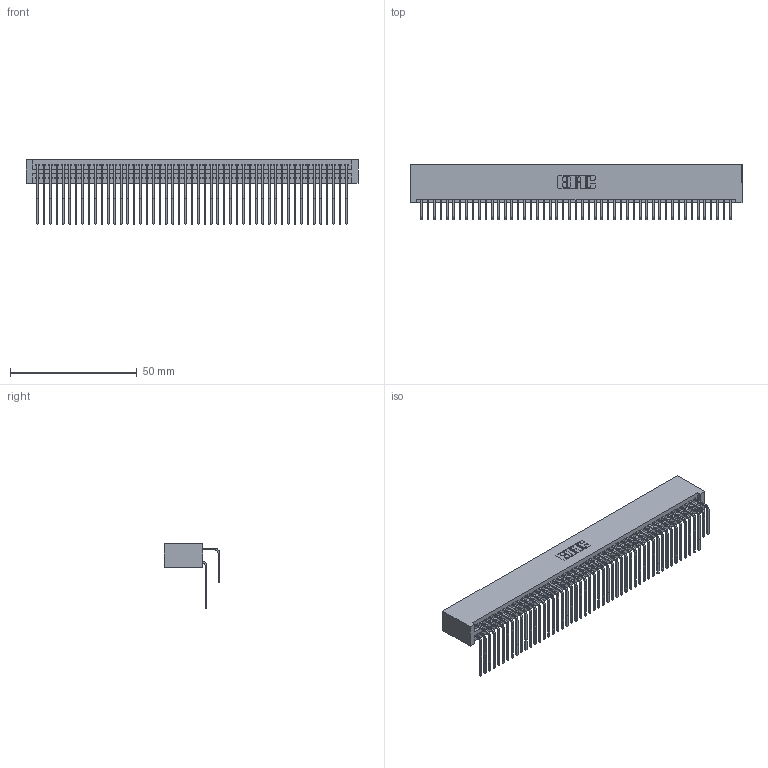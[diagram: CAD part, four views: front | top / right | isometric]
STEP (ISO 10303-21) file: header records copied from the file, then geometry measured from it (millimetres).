
FILE_DESCRIPTION (( 'STEP AP203' ), '1' );
FILE_NAME ('345-098-558-201.STEP', '2019-11-02T12:53:45', ( '' ), ( '' ), 'SwSTEP 2.0', 'SolidWorks 2016', '' );
FILE_SCHEMA (( 'CONFIG_CONTROL_DESIGN' ));
Length unit declared in the file: inch
Products named in the file (4): 345-292-001_558 Tail - 2; 345 Part_No Mounting Lugs; 345-292-001_558 559 Tail - 1; 345-098-558-201
Assembly tree (99 placements, depth 2):
  345-098-558-201
    345 Part_No Mounting Lugs
    345-292-001_558 559 Tail - 1  x49
    345-292-001_558 Tail - 2  x49
Bounding box: 131.06 x 21.83 x 25.53 mm (x, y, z)
Volume: 13977.9 mm3; surface area: 23758.9 mm2
Topology: 99 solids, 99 shells, 5214 faces, 15507 edges, 10206 vertices
Faces by surface type: plane 3506, cylinder 1708
Entity records: 38879 total; most frequent: CARTESIAN_POINT 6555, ORIENTED_EDGE 6438, DIRECTION 5739, EDGE_CURVE 3219, VECTOR 2859, LINE 2859, VERTEX_POINT 2142, AXIS2_PLACEMENT_3D 1440
